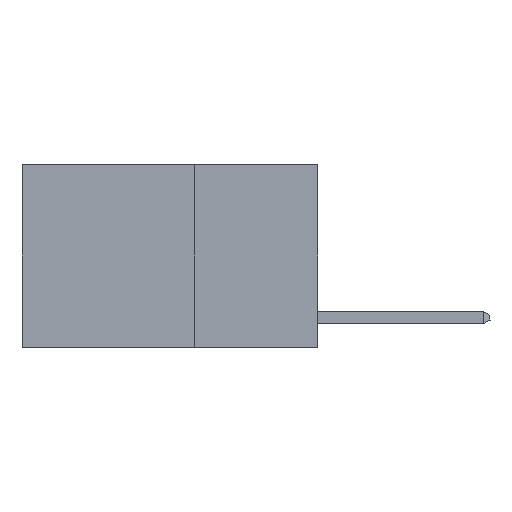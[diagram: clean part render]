
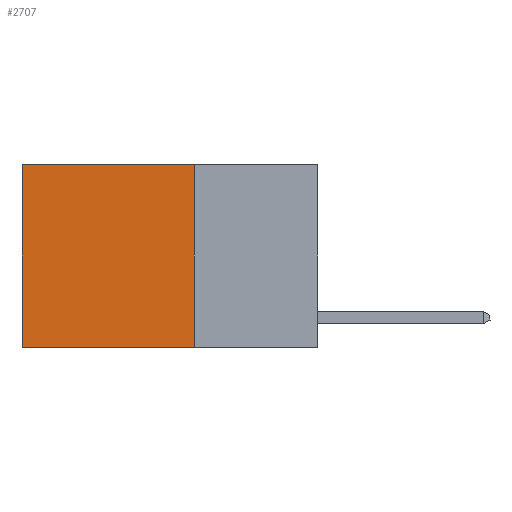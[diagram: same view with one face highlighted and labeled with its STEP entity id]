
A CAD part, left-side view. The second image highlights one B-rep face of the part: STEP entity #2707.
In plain terms, the highlighted planar face has unit normal (-1, 0, 0).
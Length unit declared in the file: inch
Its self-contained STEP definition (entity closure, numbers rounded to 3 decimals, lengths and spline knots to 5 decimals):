
#394 = CARTESIAN_POINT ( 'NONE',  ( 0.2625, 0.25, 0. ) ) ;
#721 = VECTOR ( 'NONE', #15188, 39.37008 ) ;
#1119 = ORIENTED_EDGE ( 'NONE', *, *, #13538, .T. ) ;
#1188 = AXIS2_PLACEMENT_3D ( 'NONE', #13656, #15326, #5271 ) ;
#1733 = CARTESIAN_POINT ( 'NONE',  ( 0.2625, 0.6, 0. ) ) ;
#1877 = PLANE ( 'NONE',  #1188 ) ;
#2122 = DIRECTION ( 'NONE',  ( 0., 1., 0. ) ) ;
#2301 = VERTEX_POINT ( 'NONE', #2490 ) ;
#2490 = CARTESIAN_POINT ( 'NONE',  ( 0.2625, 0.25, 0. ) ) ;
#2707 = ADVANCED_FACE ( 'NONE', ( #21396 ), #1877, .F. ) ;
#3793 = ORIENTED_EDGE ( 'NONE', *, *, #21562, .F. ) ;
#4003 = VERTEX_POINT ( 'NONE', #20470 ) ;
#4180 = VERTEX_POINT ( 'NONE', #19216 ) ;
#5126 = DIRECTION ( 'NONE',  ( 0., 0., -1. ) ) ;
#5243 = LINE ( 'NONE', #16809, #721 ) ;
#5271 = DIRECTION ( 'NONE',  ( 0., 0., -1. ) ) ;
#5694 = LINE ( 'NONE', #10997, #9644 ) ;
#7156 = LINE ( 'NONE', #394, #15538 ) ;
#7883 = EDGE_CURVE ( 'NONE', #4180, #4003, #5243, .T. ) ;
#8691 = CARTESIAN_POINT ( 'NONE',  ( 0.2625, 0.6, 0. ) ) ;
#9644 = VECTOR ( 'NONE', #12708, 39.37008 ) ;
#10997 = CARTESIAN_POINT ( 'NONE',  ( 0.2625, 0.25, 0. ) ) ;
#11814 = ORIENTED_EDGE ( 'NONE', *, *, #18248, .T. ) ;
#12072 = EDGE_LOOP ( 'NONE', ( #11814, #21086, #3793, #1119 ) ) ;
#12708 = DIRECTION ( 'NONE',  ( 0., 0., -1. ) ) ;
#13486 = VERTEX_POINT ( 'NONE', #8691 ) ;
#13538 = EDGE_CURVE ( 'NONE', #2301, #13486, #7156, .T. ) ;
#13656 = CARTESIAN_POINT ( 'NONE',  ( 0.2625, 0.25, 0. ) ) ;
#15188 = DIRECTION ( 'NONE',  ( 0., 1., 0. ) ) ;
#15326 = DIRECTION ( 'NONE',  ( 1., 0., 0. ) ) ;
#15538 = VECTOR ( 'NONE', #2122, 39.37008 ) ;
#16809 = CARTESIAN_POINT ( 'NONE',  ( 0.2625, 0.25, -0.37 ) ) ;
#17065 = VECTOR ( 'NONE', #5126, 39.37008 ) ;
#17578 = LINE ( 'NONE', #1733, #17065 ) ;
#18248 = EDGE_CURVE ( 'NONE', #13486, #4003, #17578, .T. ) ;
#19216 = CARTESIAN_POINT ( 'NONE',  ( 0.2625, 0.25, -0.37 ) ) ;
#20470 = CARTESIAN_POINT ( 'NONE',  ( 0.2625, 0.6, -0.37 ) ) ;
#21086 = ORIENTED_EDGE ( 'NONE', *, *, #7883, .F. ) ;
#21396 = FACE_OUTER_BOUND ( 'NONE', #12072, .T. ) ;
#21562 = EDGE_CURVE ( 'NONE', #2301, #4180, #5694, .T. ) ;
